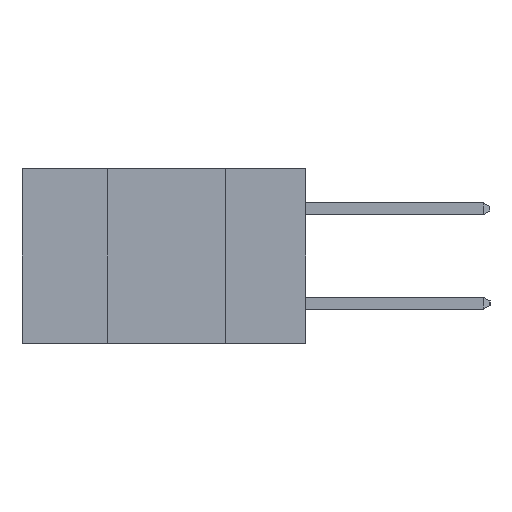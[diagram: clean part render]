
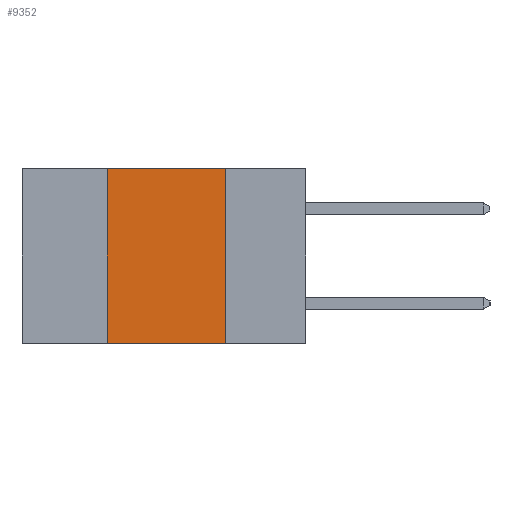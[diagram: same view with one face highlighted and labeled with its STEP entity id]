
A CAD part, left-side view. The second image highlights one B-rep face of the part: STEP entity #9352.
In plain terms, the highlighted planar face has unit normal (-1, 0, 0).
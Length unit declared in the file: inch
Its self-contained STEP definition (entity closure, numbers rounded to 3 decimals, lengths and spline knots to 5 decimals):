
#101 = VECTOR ( 'NONE', #2643, 39.37008 ) ;
#104 = ORIENTED_EDGE ( 'NONE', *, *, #2873, .F. ) ;
#2426 = ORIENTED_EDGE ( 'NONE', *, *, #7381, .F. ) ;
#2495 = CARTESIAN_POINT ( 'NONE',  ( 0., 0.17, -0.37 ) ) ;
#2643 = DIRECTION ( 'NONE',  ( 0., 0., 1. ) ) ;
#2669 = CARTESIAN_POINT ( 'NONE',  ( 0., 0.42, -0.37 ) ) ;
#2873 = EDGE_CURVE ( 'NONE', #11593, #7394, #11508, .T. ) ;
#2902 = CARTESIAN_POINT ( 'NONE',  ( 0., 0.42, -0.37 ) ) ;
#3309 = PLANE ( 'NONE',  #3827 ) ;
#3827 = AXIS2_PLACEMENT_3D ( 'NONE', #16734, #6710, #18449 ) ;
#4519 = VECTOR ( 'NONE', #7357, 39.37008 ) ;
#6710 = DIRECTION ( 'NONE',  ( 1., 0., 0. ) ) ;
#6973 = DIRECTION ( 'NONE',  ( 0., 0., -1. ) ) ;
#7357 = DIRECTION ( 'NONE',  ( 0., -1., 0. ) ) ;
#7381 = EDGE_CURVE ( 'NONE', #16221, #17191, #18021, .T. ) ;
#7394 = VERTEX_POINT ( 'NONE', #2495 ) ;
#8931 = CARTESIAN_POINT ( 'NONE',  ( 0., 0.17, -0.37 ) ) ;
#9352 = ADVANCED_FACE ( 'NONE', ( #14220 ), #3309, .F. ) ;
#9604 = EDGE_CURVE ( 'NONE', #17191, #11593, #17910, .T. ) ;
#10417 = EDGE_LOOP ( 'NONE', ( #104, #15755, #2426, #16540 ) ) ;
#11508 = LINE ( 'NONE', #8931, #16018 ) ;
#11593 = VERTEX_POINT ( 'NONE', #12034 ) ;
#12034 = CARTESIAN_POINT ( 'NONE',  ( 0., 0.17, 0. ) ) ;
#14220 = FACE_OUTER_BOUND ( 'NONE', #10417, .T. ) ;
#14241 = LINE ( 'NONE', #17084, #18727 ) ;
#15461 = CARTESIAN_POINT ( 'NONE',  ( 0., 0.42, 0. ) ) ;
#15680 = CARTESIAN_POINT ( 'NONE',  ( 0., 0.6, 0. ) ) ;
#15755 = ORIENTED_EDGE ( 'NONE', *, *, #9604, .F. ) ;
#16018 = VECTOR ( 'NONE', #6973, 39.37008 ) ;
#16221 = VERTEX_POINT ( 'NONE', #2902 ) ;
#16540 = ORIENTED_EDGE ( 'NONE', *, *, #19722, .T. ) ;
#16734 = CARTESIAN_POINT ( 'NONE',  ( 0., 0.6, 0. ) ) ;
#17084 = CARTESIAN_POINT ( 'NONE',  ( 0., 0.6, -0.37 ) ) ;
#17191 = VERTEX_POINT ( 'NONE', #15461 ) ;
#17910 = LINE ( 'NONE', #15680, #4519 ) ;
#18021 = LINE ( 'NONE', #2669, #101 ) ;
#18449 = DIRECTION ( 'NONE',  ( 0., 0., -1. ) ) ;
#18727 = VECTOR ( 'NONE', #18800, 39.37008 ) ;
#18800 = DIRECTION ( 'NONE',  ( 0., -1., 0. ) ) ;
#19722 = EDGE_CURVE ( 'NONE', #16221, #7394, #14241, .T. ) ;
